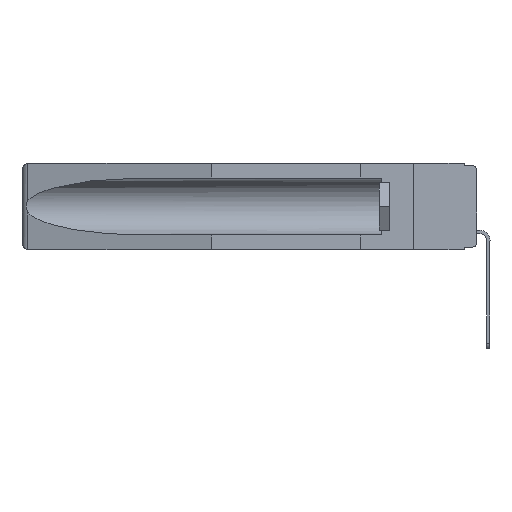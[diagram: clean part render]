
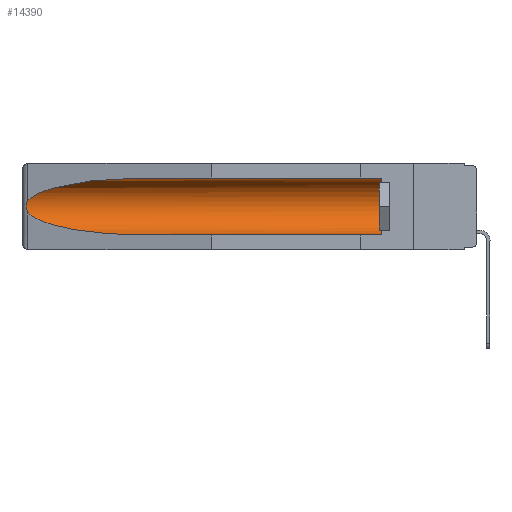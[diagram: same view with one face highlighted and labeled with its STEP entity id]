
A CAD part, left-side view. The second image highlights one B-rep face of the part: STEP entity #14390.
In plain terms, the highlighted cylindrical face has radius 2.857 mm (diameter 5.715 mm), a partial arc.
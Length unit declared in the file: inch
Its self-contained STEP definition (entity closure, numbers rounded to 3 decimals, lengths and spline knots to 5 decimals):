
#570 =( BOUNDED_CURVE ( )  B_SPLINE_CURVE ( 3, ( #8529, #1188, #11499, #14613 ),
 .UNSPECIFIED., .F., .F. ) 
 B_SPLINE_CURVE_WITH_KNOTS ( ( 4, 4 ),
 ( 4.71239, 6.08839 ),
 .UNSPECIFIED. ) 
 CURVE ( )  GEOMETRIC_REPRESENTATION_ITEM ( )  RATIONAL_B_SPLINE_CURVE ( ( 1., 0.848, 0.848, 1. ) ) 
 REPRESENTATION_ITEM ( '' )  );
#838 = ORIENTED_EDGE ( 'NONE', *, *, #2465, .F. ) ;
#1006 = LINE ( 'NONE', #1741, #12785 ) ;
#1188 = CARTESIAN_POINT ( 'NONE',  ( 0.21114, 1.30732, -0.059 ) ) ;
#1265 = FACE_OUTER_BOUND ( 'NONE', #18910, .T. ) ;
#1320 = CARTESIAN_POINT ( 'NONE',  ( 0.155, -0.30754, -0.1715 ) ) ;
#1420 = CARTESIAN_POINT ( 'NONE',  ( 0.155, 0.126, -0.1715 ) ) ;
#1741 = CARTESIAN_POINT ( 'NONE',  ( 0.155, -0.30754, -0.284 ) ) ;
#2050 = CARTESIAN_POINT ( 'NONE',  ( 0.26537, 1.52718, -0.19328 ) ) ;
#2465 = EDGE_CURVE ( 'NONE', #4393, #9806, #1006, .T. ) ;
#2962 = CARTESIAN_POINT ( 'NONE',  ( 0.155, 1.07973, -0.284 ) ) ;
#3520 = EDGE_CURVE ( 'NONE', #7522, #10747, #12996, .T. ) ;
#4335 = ORIENTED_EDGE ( 'NONE', *, *, #3520, .T. ) ;
#4393 = VERTEX_POINT ( 'NONE', #17085 ) ;
#5066 = CARTESIAN_POINT ( 'NONE',  ( 0.2673, 1.53269, -0.17917 ) ) ;
#5077 = CARTESIAN_POINT ( 'NONE',  ( 0.25451, 1.48313, -0.24835 ) ) ;
#5196 = CARTESIAN_POINT ( 'NONE',  ( 0.26654, 1.53092, -0.15636 ) ) ;
#5269 =( BOUNDED_CURVE ( )  B_SPLINE_CURVE ( 3, ( #2050, #5077, #18519, #10996 ),
 .UNSPECIFIED., .F., .F. ) 
 B_SPLINE_CURVE_WITH_KNOTS ( ( 4, 4 ),
 ( 0.1948, 1.5708 ),
 .UNSPECIFIED. ) 
 CURVE ( )  GEOMETRIC_REPRESENTATION_ITEM ( )  RATIONAL_B_SPLINE_CURVE ( ( 1., 0.848, 0.848, 1. ) ) 
 REPRESENTATION_ITEM ( '' )  );
#6008 = AXIS2_PLACEMENT_3D ( 'NONE', #1320, #13366, #17774 ) ;
#6593 = CARTESIAN_POINT ( 'NONE',  ( 0.26655, 1.53094, -0.18657 ) ) ;
#6721 = CARTESIAN_POINT ( 'NONE',  ( 0.2673, 1.5327, -0.16383 ) ) ;
#6841 = EDGE_CURVE ( 'NONE', #7728, #6927, #11926, .T. ) ;
#6927 = VERTEX_POINT ( 'NONE', #7804 ) ;
#6998 = VECTOR ( 'NONE', #12368, 39.37008 ) ;
#7178 = CYLINDRICAL_SURFACE ( 'NONE', #6008, 0.1125 ) ;
#7522 = VERTEX_POINT ( 'NONE', #10558 ) ;
#7728 = VERTEX_POINT ( 'NONE', #16698 ) ;
#7804 = CARTESIAN_POINT ( 'NONE',  ( 0.155, 1.07973, -0.059 ) ) ;
#8004 = CARTESIAN_POINT ( 'NONE',  ( 0.2675, 1.53308, -0.17534 ) ) ;
#8529 = CARTESIAN_POINT ( 'NONE',  ( 0.155, 1.07973, -0.059 ) ) ;
#9648 = CARTESIAN_POINT ( 'NONE',  ( 0.26537, 1.52718, -0.19328 ) ) ;
#9732 = CARTESIAN_POINT ( 'NONE',  ( 0.26537, 1.52718, -0.19328 ) ) ;
#9806 = VERTEX_POINT ( 'NONE', #2962 ) ;
#10227 = DIRECTION ( 'NONE',  ( 0., -1., 0. ) ) ;
#10539 = ORIENTED_EDGE ( 'NONE', *, *, #17314, .T. ) ;
#10558 = CARTESIAN_POINT ( 'NONE',  ( 0.26537, 1.52718, -0.14972 ) ) ;
#10747 = VERTEX_POINT ( 'NONE', #9648 ) ;
#10996 = CARTESIAN_POINT ( 'NONE',  ( 0.155, 1.07973, -0.284 ) ) ;
#11499 = CARTESIAN_POINT ( 'NONE',  ( 0.25451, 1.48313, -0.09465 ) ) ;
#11568 = ORIENTED_EDGE ( 'NONE', *, *, #18323, .T. ) ;
#11700 = ORIENTED_EDGE ( 'NONE', *, *, #16430, .T. ) ;
#11926 = LINE ( 'NONE', #12166, #6998 ) ;
#12166 = CARTESIAN_POINT ( 'NONE',  ( 0.155, -0.30754, -0.059 ) ) ;
#12262 = DIRECTION ( 'NONE',  ( 0., 1., 0. ) ) ;
#12368 = DIRECTION ( 'NONE',  ( 0., 1., 0. ) ) ;
#12785 = VECTOR ( 'NONE', #12262, 39.37008 ) ;
#12996 = B_SPLINE_CURVE_WITH_KNOTS ( 'NONE', 3,
 ( #15603, #18700, #5196, #6721, #14031, #8004, #5066, #6593, #17132, #9732 ),
 .UNSPECIFIED., .F., .F.,
 ( 4, 2, 2, 2, 4 ),
 ( 0., 0.00029, 0.00058, 0.00087, 0.00117 ),
 .UNSPECIFIED. ) ;
#13366 = DIRECTION ( 'NONE',  ( 0., 1., 0. ) ) ;
#13483 = CIRCLE ( 'NONE', #19299, 0.1125 ) ;
#14031 = CARTESIAN_POINT ( 'NONE',  ( 0.2675, 1.53308, -0.16763 ) ) ;
#14390 = ADVANCED_FACE ( 'NONE', ( #1265 ), #7178, .F. ) ;
#14613 = CARTESIAN_POINT ( 'NONE',  ( 0.26537, 1.52718, -0.14972 ) ) ;
#15603 = CARTESIAN_POINT ( 'NONE',  ( 0.26537, 1.52718, -0.14972 ) ) ;
#16430 = EDGE_CURVE ( 'NONE', #10747, #9806, #5269, .T. ) ;
#16698 = CARTESIAN_POINT ( 'NONE',  ( 0.155, 0.126, -0.059 ) ) ;
#17085 = CARTESIAN_POINT ( 'NONE',  ( 0.155, 0.126, -0.284 ) ) ;
#17132 = CARTESIAN_POINT ( 'NONE',  ( 0.26597, 1.5296, -0.19026 ) ) ;
#17314 = EDGE_CURVE ( 'NONE', #4393, #7728, #13483, .T. ) ;
#17774 = DIRECTION ( 'NONE',  ( 0., 0., 1. ) ) ;
#17937 = DIRECTION ( 'NONE',  ( 0., 0., 1. ) ) ;
#18316 = ORIENTED_EDGE ( 'NONE', *, *, #6841, .T. ) ;
#18323 = EDGE_CURVE ( 'NONE', #6927, #7522, #570, .T. ) ;
#18519 = CARTESIAN_POINT ( 'NONE',  ( 0.21114, 1.30732, -0.284 ) ) ;
#18700 = CARTESIAN_POINT ( 'NONE',  ( 0.26597, 1.52961, -0.15275 ) ) ;
#18910 = EDGE_LOOP ( 'NONE', ( #11568, #4335, #11700, #838, #10539, #18316 ) ) ;
#19299 = AXIS2_PLACEMENT_3D ( 'NONE', #1420, #10227, #17937 ) ;
